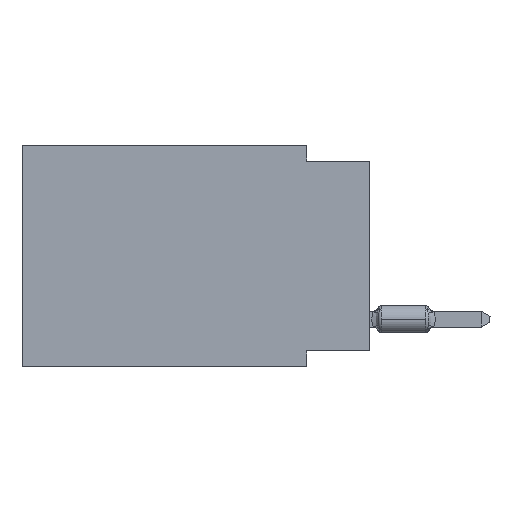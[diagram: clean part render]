
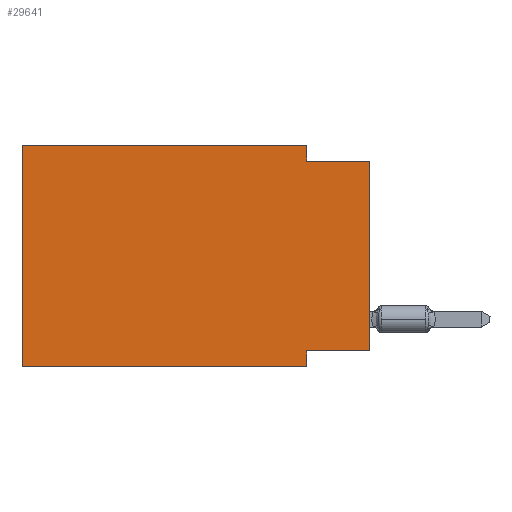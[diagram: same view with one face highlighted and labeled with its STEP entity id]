
A CAD part, left-side view. The second image highlights one B-rep face of the part: STEP entity #29641.
In plain terms, the highlighted planar face has unit normal (-1, 0, 0).
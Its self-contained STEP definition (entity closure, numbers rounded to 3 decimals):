
#178 = EDGE_CURVE ( 'NONE', #23707, #15213, #17307, .T. ) ;
#462 = LINE ( 'NONE', #32821, #12163 ) ;
#1639 = VERTEX_POINT ( 'NONE', #12975 ) ;
#1806 = CARTESIAN_POINT ( 'NONE',  ( 0., 0., -8.255 ) ) ;
#2055 = VERTEX_POINT ( 'NONE', #20424 ) ;
#2267 = LINE ( 'NONE', #17435, #17570 ) ;
#3772 = DIRECTION ( 'NONE',  ( 0., 0., -1. ) ) ;
#5319 = DIRECTION ( 'NONE',  ( 0., -1., 0. ) ) ;
#5714 = EDGE_CURVE ( 'NONE', #2055, #19107, #10002, .T. ) ;
#6221 = ORIENTED_EDGE ( 'NONE', *, *, #32013, .F. ) ;
#6433 = LINE ( 'NONE', #8407, #9723 ) ;
#6495 = EDGE_CURVE ( 'NONE', #19107, #18840, #32613, .T. ) ;
#7215 = VERTEX_POINT ( 'NONE', #20232 ) ;
#7589 = EDGE_CURVE ( 'NONE', #2055, #7215, #462, .T. ) ;
#8407 = CARTESIAN_POINT ( 'NONE',  ( 0., 2.54, 0. ) ) ;
#8819 = DIRECTION ( 'NONE',  ( 0., 0., 1. ) ) ;
#9097 = AXIS2_PLACEMENT_3D ( 'NONE', #11935, #22084, #3772 ) ;
#9482 = DIRECTION ( 'NONE',  ( 0., 0., 1. ) ) ;
#9723 = VECTOR ( 'NONE', #13932, 1000. ) ;
#9731 = VERTEX_POINT ( 'NONE', #13238 ) ;
#10002 = LINE ( 'NONE', #30355, #29116 ) ;
#11547 = VECTOR ( 'NONE', #9482, 1000. ) ;
#11935 = CARTESIAN_POINT ( 'NONE',  ( 0., 13.97, 0. ) ) ;
#12163 = VECTOR ( 'NONE', #5319, 1000. ) ;
#12849 = CARTESIAN_POINT ( 'NONE',  ( 0., 0., -0.635 ) ) ;
#12876 = EDGE_CURVE ( 'NONE', #23707, #9731, #31877, .T. ) ;
#12975 = CARTESIAN_POINT ( 'NONE',  ( 0., 2.54, -0.635 ) ) ;
#13238 = CARTESIAN_POINT ( 'NONE',  ( 0., 2.54, -8.255 ) ) ;
#13754 = DIRECTION ( 'NONE',  ( 0., -1., 0. ) ) ;
#13932 = DIRECTION ( 'NONE',  ( 0., 0., -1. ) ) ;
#14088 = CARTESIAN_POINT ( 'NONE',  ( 0., 0., -0.635 ) ) ;
#14095 = PLANE ( 'NONE',  #9097 ) ;
#15213 = VERTEX_POINT ( 'NONE', #12849 ) ;
#15412 = ORIENTED_EDGE ( 'NONE', *, *, #5714, .F. ) ;
#16239 = EDGE_LOOP ( 'NONE', ( #28828, #6221, #27235, #30942, #15412, #26414, #21728, #28672 ) ) ;
#16254 = LINE ( 'NONE', #14088, #22485 ) ;
#16601 = CARTESIAN_POINT ( 'NONE',  ( 0., 2.54, 0. ) ) ;
#17307 = LINE ( 'NONE', #30312, #11547 ) ;
#17435 = CARTESIAN_POINT ( 'NONE',  ( 0., 2.54, -8.89 ) ) ;
#17535 = VECTOR ( 'NONE', #31093, 1000. ) ;
#17570 = VECTOR ( 'NONE', #32304, 1000. ) ;
#18593 = EDGE_CURVE ( 'NONE', #9731, #7215, #2267, .T. ) ;
#18840 = VERTEX_POINT ( 'NONE', #16601 ) ;
#19107 = VERTEX_POINT ( 'NONE', #26051 ) ;
#20232 = CARTESIAN_POINT ( 'NONE',  ( 0., 2.54, -8.89 ) ) ;
#20424 = CARTESIAN_POINT ( 'NONE',  ( 0., 13.97, -8.89 ) ) ;
#20568 = CARTESIAN_POINT ( 'NONE',  ( 0., 0., -8.255 ) ) ;
#21728 = ORIENTED_EDGE ( 'NONE', *, *, #18593, .F. ) ;
#22084 = DIRECTION ( 'NONE',  ( 1., 0., 0. ) ) ;
#22485 = VECTOR ( 'NONE', #13754, 1000. ) ;
#23079 = CARTESIAN_POINT ( 'NONE',  ( 0., 13.97, 0. ) ) ;
#23707 = VERTEX_POINT ( 'NONE', #1806 ) ;
#25502 = VECTOR ( 'NONE', #27780, 1000. ) ;
#26051 = CARTESIAN_POINT ( 'NONE',  ( 0., 13.97, 0. ) ) ;
#26414 = ORIENTED_EDGE ( 'NONE', *, *, #7589, .T. ) ;
#27235 = ORIENTED_EDGE ( 'NONE', *, *, #31890, .F. ) ;
#27780 = DIRECTION ( 'NONE',  ( 0., -1., 0. ) ) ;
#28672 = ORIENTED_EDGE ( 'NONE', *, *, #12876, .F. ) ;
#28828 = ORIENTED_EDGE ( 'NONE', *, *, #178, .T. ) ;
#29116 = VECTOR ( 'NONE', #8819, 1000. ) ;
#29280 = FACE_OUTER_BOUND ( 'NONE', #16239, .T. ) ;
#29641 = ADVANCED_FACE ( 'NONE', ( #29280 ), #14095, .F. ) ;
#30312 = CARTESIAN_POINT ( 'NONE',  ( 0., 0., 0. ) ) ;
#30355 = CARTESIAN_POINT ( 'NONE',  ( 0., 13.97, 0. ) ) ;
#30942 = ORIENTED_EDGE ( 'NONE', *, *, #6495, .F. ) ;
#31093 = DIRECTION ( 'NONE',  ( 0., 1., 0. ) ) ;
#31877 = LINE ( 'NONE', #20568, #17535 ) ;
#31890 = EDGE_CURVE ( 'NONE', #18840, #1639, #6433, .T. ) ;
#32013 = EDGE_CURVE ( 'NONE', #1639, #15213, #16254, .T. ) ;
#32304 = DIRECTION ( 'NONE',  ( 0., 0., -1. ) ) ;
#32613 = LINE ( 'NONE', #23079, #25502 ) ;
#32821 = CARTESIAN_POINT ( 'NONE',  ( 0., 13.97, -8.89 ) ) ;
